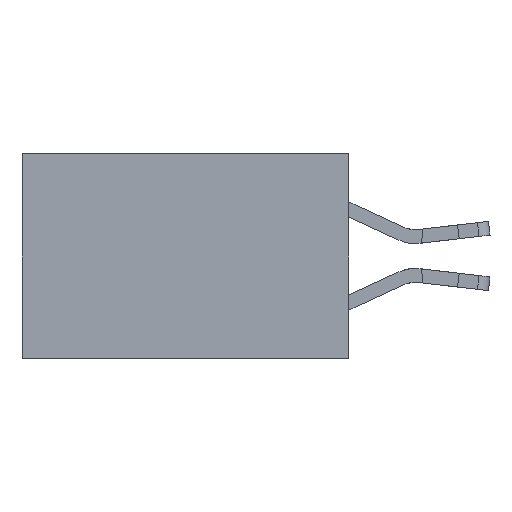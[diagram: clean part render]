
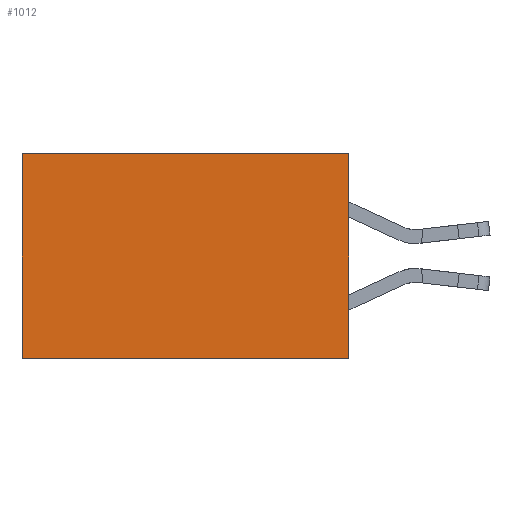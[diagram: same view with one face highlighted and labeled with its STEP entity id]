
A CAD part, left-side view. The second image highlights one B-rep face of the part: STEP entity #1012.
In plain terms, the highlighted planar face has unit normal (-1, 0, 0).
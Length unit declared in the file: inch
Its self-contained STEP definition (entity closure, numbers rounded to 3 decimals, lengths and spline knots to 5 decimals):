
#1012 = ADVANCED_FACE ( 'NONE', ( #12592 ), #19596, .F. ) ;
#1863 = VERTEX_POINT ( 'NONE', #7354 ) ;
#2081 = ORIENTED_EDGE ( 'NONE', *, *, #4866, .F. ) ;
#2137 = VECTOR ( 'NONE', #5154, 39.37008 ) ;
#2392 = DIRECTION ( 'NONE',  ( 0., 0., -1. ) ) ;
#2408 = EDGE_CURVE ( 'NONE', #8657, #1863, #4119, .T. ) ;
#2642 = AXIS2_PLACEMENT_3D ( 'NONE', #8156, #4891, #2392 ) ;
#2706 = LINE ( 'NONE', #19363, #2137 ) ;
#3004 = DIRECTION ( 'NONE',  ( 0., 1., 0. ) ) ;
#3465 = EDGE_CURVE ( 'NONE', #17001, #14108, #15011, .T. ) ;
#3970 = CARTESIAN_POINT ( 'NONE',  ( 0.277, 0., -0.37 ) ) ;
#4119 = LINE ( 'NONE', #17510, #17264 ) ;
#4866 = EDGE_CURVE ( 'NONE', #8657, #17001, #14950, .T. ) ;
#4891 = DIRECTION ( 'NONE',  ( 1., 0., 0. ) ) ;
#5154 = DIRECTION ( 'NONE',  ( 0., 0., -1. ) ) ;
#6055 = CARTESIAN_POINT ( 'NONE',  ( 0.277, 0.59, -0.37 ) ) ;
#7354 = CARTESIAN_POINT ( 'NONE',  ( 0.277, 0.59, 0. ) ) ;
#8156 = CARTESIAN_POINT ( 'NONE',  ( 0.277, 0., -0.37 ) ) ;
#8657 = VERTEX_POINT ( 'NONE', #19310 ) ;
#9484 = ORIENTED_EDGE ( 'NONE', *, *, #15125, .T. ) ;
#12435 = ORIENTED_EDGE ( 'NONE', *, *, #2408, .T. ) ;
#12592 = FACE_OUTER_BOUND ( 'NONE', #20764, .T. ) ;
#14108 = VERTEX_POINT ( 'NONE', #6055 ) ;
#14216 = DIRECTION ( 'NONE',  ( 0., 1., 0. ) ) ;
#14844 = CARTESIAN_POINT ( 'NONE',  ( 0.277, 0., -0.37 ) ) ;
#14950 = LINE ( 'NONE', #21368, #18524 ) ;
#15011 = LINE ( 'NONE', #14844, #19109 ) ;
#15125 = EDGE_CURVE ( 'NONE', #1863, #14108, #2706, .T. ) ;
#17001 = VERTEX_POINT ( 'NONE', #3970 ) ;
#17264 = VECTOR ( 'NONE', #14216, 39.37008 ) ;
#17510 = CARTESIAN_POINT ( 'NONE',  ( 0.277, 0., 0. ) ) ;
#18524 = VECTOR ( 'NONE', #21601, 39.37008 ) ;
#19109 = VECTOR ( 'NONE', #3004, 39.37008 ) ;
#19310 = CARTESIAN_POINT ( 'NONE',  ( 0.277, 0., 0. ) ) ;
#19363 = CARTESIAN_POINT ( 'NONE',  ( 0.277, 0.59, -0.37 ) ) ;
#19596 = PLANE ( 'NONE',  #2642 ) ;
#20764 = EDGE_LOOP ( 'NONE', ( #9484, #21850, #2081, #12435 ) ) ;
#21368 = CARTESIAN_POINT ( 'NONE',  ( 0.277, 0., -0.37 ) ) ;
#21601 = DIRECTION ( 'NONE',  ( 0., 0., -1. ) ) ;
#21850 = ORIENTED_EDGE ( 'NONE', *, *, #3465, .F. ) ;
